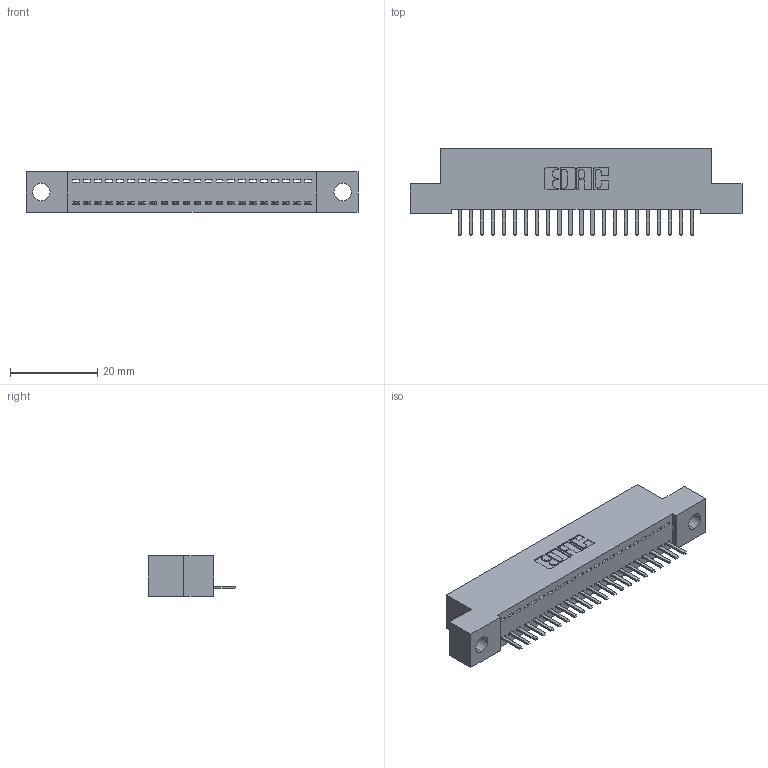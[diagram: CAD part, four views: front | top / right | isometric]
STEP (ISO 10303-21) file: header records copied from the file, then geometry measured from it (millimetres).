
FILE_DESCRIPTION (( 'STEP AP203' ), '1' );
FILE_NAME ('342-022-520-104.STEP', '2018-08-11T00:10:39', ( '' ), ( '' ), 'SwSTEP 2.0', 'SolidWorks 2016', '' );
FILE_SCHEMA (( 'CONFIG_CONTROL_DESIGN' ));
Length unit declared in the file: inch
Products named in the file (3): 342-022-520-104; 342 Part_.156 TH; 345-292-001_345-293-120
Assembly tree (23 placements, depth 2):
  342-022-520-104
    342 Part_.156 TH
    345-292-001_345-293-120  x22
Bounding box: 76.2 x 20.02 x 9.4 mm (x, y, z)
Volume: 6457.2 mm3; surface area: 8725.1 mm2
Topology: 23 solids, 23 shells, 1474 faces, 4347 edges, 2838 vertices
Faces by surface type: plane 1034, cylinder 440
Entity records: 16021 total; most frequent: CARTESIAN_POINT 2784, ORIENTED_EDGE 2730, DIRECTION 2377, EDGE_CURVE 1365, VECTOR 1233, LINE 1233, VERTEX_POINT 906, AXIS2_PLACEMENT_3D 572
